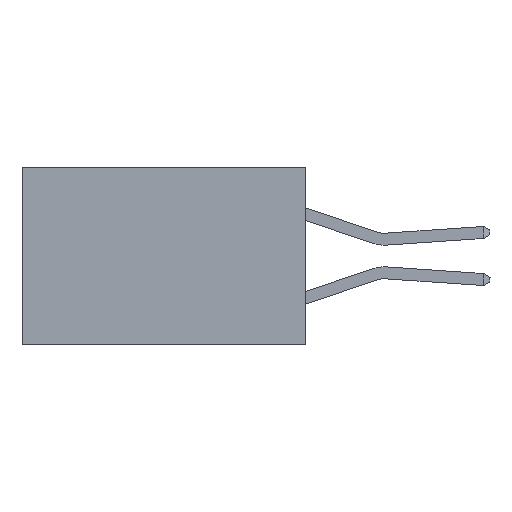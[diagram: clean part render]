
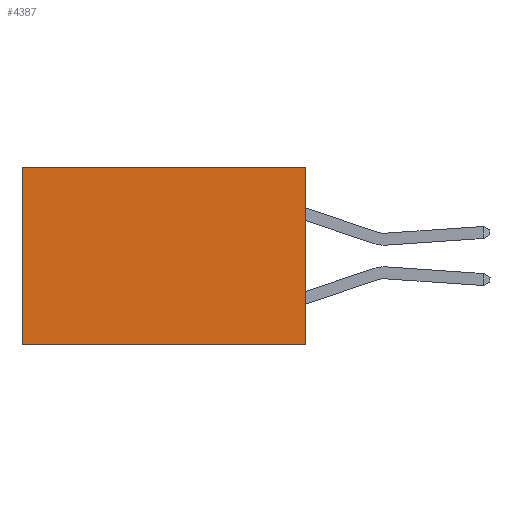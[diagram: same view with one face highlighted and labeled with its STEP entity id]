
A CAD part, left-side view. The second image highlights one B-rep face of the part: STEP entity #4387.
In plain terms, the highlighted planar face has unit normal (-1, 0, 0).
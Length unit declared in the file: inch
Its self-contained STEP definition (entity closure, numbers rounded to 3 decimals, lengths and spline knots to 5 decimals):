
#281 = CARTESIAN_POINT ( 'NONE',  ( 0.277, 0.59, -0.37 ) ) ;
#2052 = DIRECTION ( 'NONE',  ( 0., 0., -1. ) ) ;
#2133 = DIRECTION ( 'NONE',  ( 1., 0., 0. ) ) ;
#2177 = PLANE ( 'NONE',  #13320 ) ;
#2379 = DIRECTION ( 'NONE',  ( 0., 1., 0. ) ) ;
#2873 = LINE ( 'NONE', #16888, #9209 ) ;
#3213 = LINE ( 'NONE', #13092, #22007 ) ;
#4387 = ADVANCED_FACE ( 'NONE', ( #7053 ), #2177, .F. ) ;
#5138 = CARTESIAN_POINT ( 'NONE',  ( 0.277, 0., -0.37 ) ) ;
#6664 = ORIENTED_EDGE ( 'NONE', *, *, #26110, .T. ) ;
#6689 = VERTEX_POINT ( 'NONE', #10442 ) ;
#6843 = CARTESIAN_POINT ( 'NONE',  ( 0.277, 0., -0.37 ) ) ;
#7053 = FACE_OUTER_BOUND ( 'NONE', #27398, .T. ) ;
#8466 = DIRECTION ( 'NONE',  ( 0., 0., -1. ) ) ;
#9209 = VECTOR ( 'NONE', #27468, 39.37008 ) ;
#10442 = CARTESIAN_POINT ( 'NONE',  ( 0.277, 0.59, -0.37 ) ) ;
#10505 = EDGE_CURVE ( 'NONE', #13202, #6689, #2873, .T. ) ;
#11940 = DIRECTION ( 'NONE',  ( 0., 0., -1. ) ) ;
#13092 = CARTESIAN_POINT ( 'NONE',  ( 0.277, 0., 0. ) ) ;
#13202 = VERTEX_POINT ( 'NONE', #5138 ) ;
#13320 = AXIS2_PLACEMENT_3D ( 'NONE', #6843, #2133, #2052 ) ;
#13691 = VECTOR ( 'NONE', #8466, 39.37008 ) ;
#15149 = CARTESIAN_POINT ( 'NONE',  ( 0.277, 0., 0. ) ) ;
#15447 = VERTEX_POINT ( 'NONE', #15149 ) ;
#15600 = EDGE_CURVE ( 'NONE', #15447, #26140, #3213, .T. ) ;
#16888 = CARTESIAN_POINT ( 'NONE',  ( 0.277, 0., -0.37 ) ) ;
#17663 = ORIENTED_EDGE ( 'NONE', *, *, #15600, .T. ) ;
#17820 = LINE ( 'NONE', #281, #13691 ) ;
#19806 = CARTESIAN_POINT ( 'NONE',  ( 0.277, 0., -0.37 ) ) ;
#20712 = VECTOR ( 'NONE', #11940, 39.37008 ) ;
#20966 = EDGE_CURVE ( 'NONE', #15447, #13202, #21551, .T. ) ;
#21551 = LINE ( 'NONE', #19806, #20712 ) ;
#22007 = VECTOR ( 'NONE', #2379, 39.37008 ) ;
#24398 = CARTESIAN_POINT ( 'NONE',  ( 0.277, 0.59, 0. ) ) ;
#26110 = EDGE_CURVE ( 'NONE', #26140, #6689, #17820, .T. ) ;
#26140 = VERTEX_POINT ( 'NONE', #24398 ) ;
#26917 = ORIENTED_EDGE ( 'NONE', *, *, #20966, .F. ) ;
#27398 = EDGE_LOOP ( 'NONE', ( #6664, #32349, #26917, #17663 ) ) ;
#27468 = DIRECTION ( 'NONE',  ( 0., 1., 0. ) ) ;
#32349 = ORIENTED_EDGE ( 'NONE', *, *, #10505, .F. ) ;
